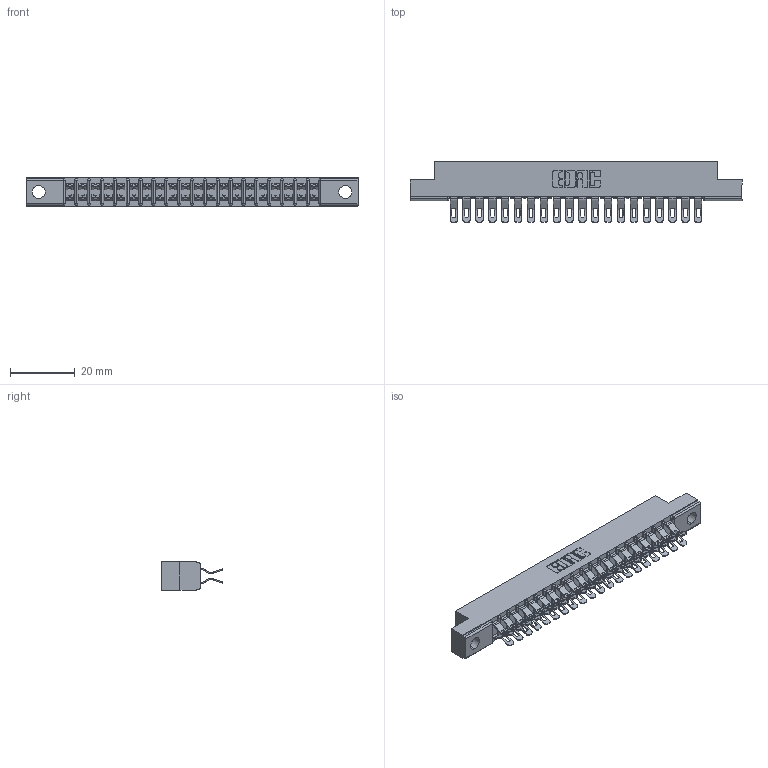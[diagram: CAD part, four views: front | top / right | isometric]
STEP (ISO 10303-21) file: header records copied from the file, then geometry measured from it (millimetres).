
FILE_DESCRIPTION (( 'STEP AP203' ), '1' );
FILE_NAME ('357-040-455-202.STEP', '2020-10-03T20:59:28', ( '' ), ( '' ), 'SwSTEP 2.0', 'SolidWorks 2020', '' );
FILE_SCHEMA (( 'CONFIG_CONTROL_DESIGN' ));
Length unit declared in the file: inch
Products named in the file (3): 357-040-455-202; 307 Part_.128 Dia Mounting Holes; 307-290-001_555
Assembly tree (41 placements, depth 2):
  357-040-455-202
    307 Part_.128 Dia Mounting Holes
    307-290-001_555  x40
Bounding box: 102.26 x 18.75 x 8.71 mm (x, y, z)
Volume: 6720.5 mm3; surface area: 12270.7 mm2
Topology: 41 solids, 41 shells, 2579 faces, 7563 edges, 4930 vertices
Faces by surface type: plane 1430, cylinder 1107, sphere 42
Entity records: 21037 total; most frequent: CARTESIAN_POINT 3452, ORIENTED_EDGE 3420, DIRECTION 3398, EDGE_CURVE 1710, VECTOR 1290, LINE 1290, VERTEX_POINT 1108, AXIS2_PLACEMENT_3D 1054
